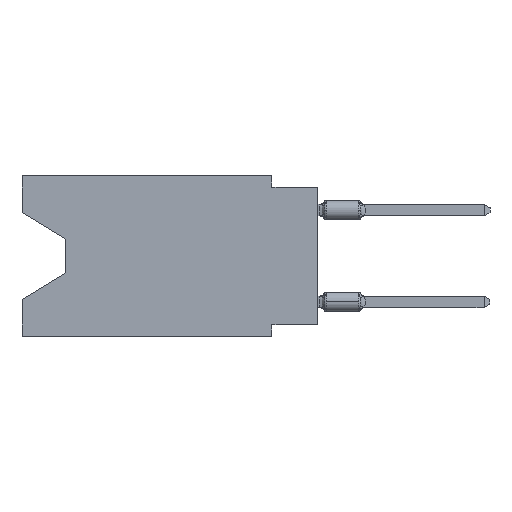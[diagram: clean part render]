
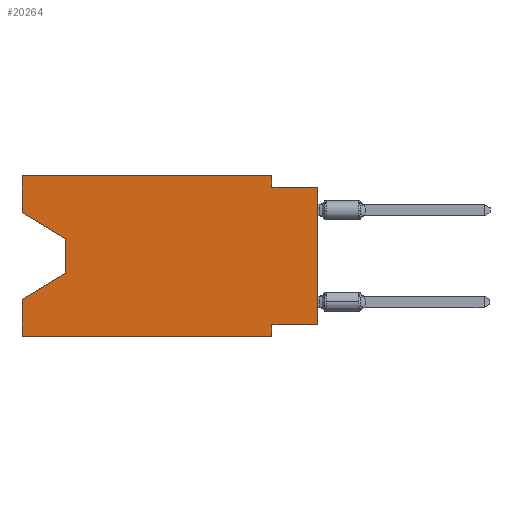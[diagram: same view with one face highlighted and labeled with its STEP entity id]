
A CAD part, left-side view. The second image highlights one B-rep face of the part: STEP entity #20264.
In plain terms, the highlighted planar face has unit normal (-1, 0, 0).
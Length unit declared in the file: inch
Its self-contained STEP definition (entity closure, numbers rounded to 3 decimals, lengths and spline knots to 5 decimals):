
#283 = DIRECTION ( 'NONE',  ( 0., 1., 0. ) ) ;
#300 = ORIENTED_EDGE ( 'NONE', *, *, #5334, .F. ) ;
#491 = LINE ( 'NONE', #8131, #3685 ) ;
#577 = DIRECTION ( 'NONE',  ( 0., 0.855, -0.519 ) ) ;
#759 = DIRECTION ( 'NONE',  ( 0., 0., -1. ) ) ;
#1188 = EDGE_CURVE ( 'NONE', #12067, #18716, #22330, .T. ) ;
#1626 = LINE ( 'NONE', #13136, #8910 ) ;
#1726 = CARTESIAN_POINT ( 'NONE',  ( 0., 0.645, 0. ) ) ;
#1903 = ORIENTED_EDGE ( 'NONE', *, *, #20522, .F. ) ;
#1996 = CARTESIAN_POINT ( 'NONE',  ( 0., 0.645, -0.35 ) ) ;
#2144 = VERTEX_POINT ( 'NONE', #23292 ) ;
#2446 = ORIENTED_EDGE ( 'NONE', *, *, #23422, .F. ) ;
#2512 = EDGE_CURVE ( 'NONE', #20390, #15809, #13897, .T. ) ;
#2544 = DIRECTION ( 'NONE',  ( 0., -1., 0. ) ) ;
#2744 = EDGE_CURVE ( 'NONE', #20390, #2144, #14390, .T. ) ;
#2841 = CARTESIAN_POINT ( 'NONE',  ( 0., 0.1, -0.325 ) ) ;
#2979 = CARTESIAN_POINT ( 'NONE',  ( 0., 0.1, 0. ) ) ;
#3092 = VECTOR ( 'NONE', #2544, 39.37008 ) ;
#3402 = ORIENTED_EDGE ( 'NONE', *, *, #6269, .F. ) ;
#3581 = DIRECTION ( 'NONE',  ( 0., -0.855, -0.519 ) ) ;
#3617 = DIRECTION ( 'NONE',  ( 0., -1., 0. ) ) ;
#3662 = DIRECTION ( 'NONE',  ( 0., -1., 0. ) ) ;
#3685 = VECTOR ( 'NONE', #15753, 39.37008 ) ;
#4237 = ORIENTED_EDGE ( 'NONE', *, *, #24084, .T. ) ;
#4319 = CARTESIAN_POINT ( 'NONE',  ( 0., 0.55, -0.212 ) ) ;
#4502 = VECTOR ( 'NONE', #3581, 39.37008 ) ;
#4634 = ORIENTED_EDGE ( 'NONE', *, *, #5280, .F. ) ;
#4849 = VERTEX_POINT ( 'NONE', #20904 ) ;
#5280 = EDGE_CURVE ( 'NONE', #17353, #15891, #491, .T. ) ;
#5308 = LINE ( 'NONE', #9075, #13326 ) ;
#5334 = EDGE_CURVE ( 'NONE', #19353, #7319, #1626, .T. ) ;
#5402 = CARTESIAN_POINT ( 'NONE',  ( 0., 0.55, -0.138 ) ) ;
#5715 = CARTESIAN_POINT ( 'NONE',  ( 0., 0.645, -0.26975 ) ) ;
#5813 = VECTOR ( 'NONE', #577, 39.37008 ) ;
#6269 = EDGE_CURVE ( 'NONE', #18716, #19353, #5308, .T. ) ;
#7106 = LINE ( 'NONE', #13217, #4502 ) ;
#7319 = VERTEX_POINT ( 'NONE', #23875 ) ;
#7554 = VECTOR ( 'NONE', #3617, 39.37008 ) ;
#8131 = CARTESIAN_POINT ( 'NONE',  ( 0., 0.645, 0. ) ) ;
#8150 = ORIENTED_EDGE ( 'NONE', *, *, #2744, .T. ) ;
#8525 = VECTOR ( 'NONE', #16962, 39.37008 ) ;
#8910 = VECTOR ( 'NONE', #24266, 39.37008 ) ;
#9075 = CARTESIAN_POINT ( 'NONE',  ( 0., 0.645, 0. ) ) ;
#10250 = EDGE_CURVE ( 'NONE', #21456, #19616, #22405, .T. ) ;
#10506 = CARTESIAN_POINT ( 'NONE',  ( 0., 0.645, -0.35 ) ) ;
#11517 = ORIENTED_EDGE ( 'NONE', *, *, #10250, .T. ) ;
#12067 = VERTEX_POINT ( 'NONE', #18918 ) ;
#12901 = DIRECTION ( 'NONE',  ( 0., 0., -1. ) ) ;
#13029 = DIRECTION ( 'NONE',  ( 0., 0., -1. ) ) ;
#13136 = CARTESIAN_POINT ( 'NONE',  ( 0., 0.1, 0. ) ) ;
#13217 = CARTESIAN_POINT ( 'NONE',  ( 0., 0.645, -0.08025 ) ) ;
#13326 = VECTOR ( 'NONE', #3662, 39.37008 ) ;
#13606 = CARTESIAN_POINT ( 'NONE',  ( 0., 0.55, -0.212 ) ) ;
#13650 = CARTESIAN_POINT ( 'NONE',  ( 0., 0., -0.325 ) ) ;
#13897 = LINE ( 'NONE', #13650, #14032 ) ;
#14032 = VECTOR ( 'NONE', #283, 39.37008 ) ;
#14390 = LINE ( 'NONE', #24005, #14463 ) ;
#14463 = VECTOR ( 'NONE', #22019, 39.37008 ) ;
#14771 = PLANE ( 'NONE',  #19890 ) ;
#14902 = EDGE_CURVE ( 'NONE', #12067, #21456, #7106, .T. ) ;
#15010 = LINE ( 'NONE', #1996, #7554 ) ;
#15341 = VECTOR ( 'NONE', #13029, 39.37008 ) ;
#15515 = ORIENTED_EDGE ( 'NONE', *, *, #1188, .F. ) ;
#15753 = DIRECTION ( 'NONE',  ( 0., 0., 1. ) ) ;
#15781 = CARTESIAN_POINT ( 'NONE',  ( 0., 0., -0.325 ) ) ;
#15809 = VERTEX_POINT ( 'NONE', #2841 ) ;
#15891 = VERTEX_POINT ( 'NONE', #5715 ) ;
#15955 = LINE ( 'NONE', #19700, #3092 ) ;
#16962 = DIRECTION ( 'NONE',  ( 0., 0., 1. ) ) ;
#17353 = VERTEX_POINT ( 'NONE', #10506 ) ;
#17609 = EDGE_CURVE ( 'NONE', #19616, #15891, #21455, .T. ) ;
#17776 = LINE ( 'NONE', #23744, #24273 ) ;
#18661 = DIRECTION ( 'NONE',  ( 1., 0., 0. ) ) ;
#18716 = VERTEX_POINT ( 'NONE', #1726 ) ;
#18810 = ORIENTED_EDGE ( 'NONE', *, *, #14902, .T. ) ;
#18918 = CARTESIAN_POINT ( 'NONE',  ( 0., 0.645, -0.08025 ) ) ;
#19353 = VERTEX_POINT ( 'NONE', #2979 ) ;
#19616 = VERTEX_POINT ( 'NONE', #13606 ) ;
#19700 = CARTESIAN_POINT ( 'NONE',  ( 0., 0., -0.025 ) ) ;
#19890 = AXIS2_PLACEMENT_3D ( 'NONE', #22514, #18661, #12901 ) ;
#20264 = ADVANCED_FACE ( 'NONE', ( #24390 ), #14771, .F. ) ;
#20390 = VERTEX_POINT ( 'NONE', #15781 ) ;
#20522 = EDGE_CURVE ( 'NONE', #15809, #4849, #17776, .T. ) ;
#20904 = CARTESIAN_POINT ( 'NONE',  ( 0., 0.1, -0.35 ) ) ;
#20912 = ORIENTED_EDGE ( 'NONE', *, *, #2512, .F. ) ;
#21455 = LINE ( 'NONE', #4319, #5813 ) ;
#21456 = VERTEX_POINT ( 'NONE', #23616 ) ;
#22019 = DIRECTION ( 'NONE',  ( 0., 0., 1. ) ) ;
#22330 = LINE ( 'NONE', #24442, #8525 ) ;
#22405 = LINE ( 'NONE', #5402, #15341 ) ;
#22514 = CARTESIAN_POINT ( 'NONE',  ( 0., 0.645, 0. ) ) ;
#23292 = CARTESIAN_POINT ( 'NONE',  ( 0., 0., -0.025 ) ) ;
#23422 = EDGE_CURVE ( 'NONE', #7319, #2144, #15955, .T. ) ;
#23616 = CARTESIAN_POINT ( 'NONE',  ( 0., 0.55, -0.138 ) ) ;
#23744 = CARTESIAN_POINT ( 'NONE',  ( 0., 0.1, -0.35 ) ) ;
#23875 = CARTESIAN_POINT ( 'NONE',  ( 0., 0.1, -0.025 ) ) ;
#24005 = CARTESIAN_POINT ( 'NONE',  ( 0., 0., 0. ) ) ;
#24084 = EDGE_CURVE ( 'NONE', #17353, #4849, #15010, .T. ) ;
#24231 = ORIENTED_EDGE ( 'NONE', *, *, #17609, .T. ) ;
#24266 = DIRECTION ( 'NONE',  ( 0., 0., -1. ) ) ;
#24273 = VECTOR ( 'NONE', #759, 39.37008 ) ;
#24390 = FACE_OUTER_BOUND ( 'NONE', #24700, .T. ) ;
#24442 = CARTESIAN_POINT ( 'NONE',  ( 0., 0.645, 0. ) ) ;
#24700 = EDGE_LOOP ( 'NONE', ( #18810, #11517, #24231, #4634, #4237, #1903, #20912, #8150, #2446, #300, #3402, #15515 ) ) ;
